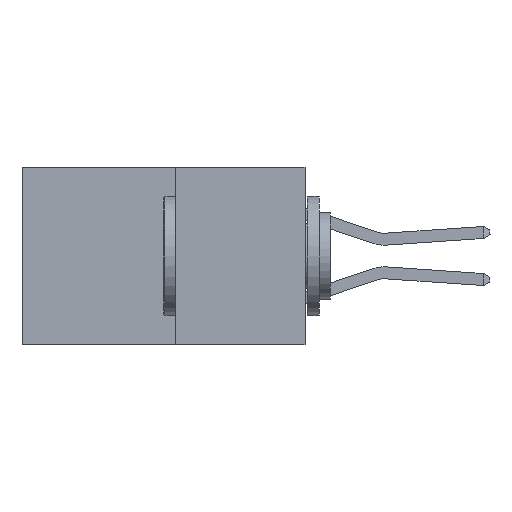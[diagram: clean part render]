
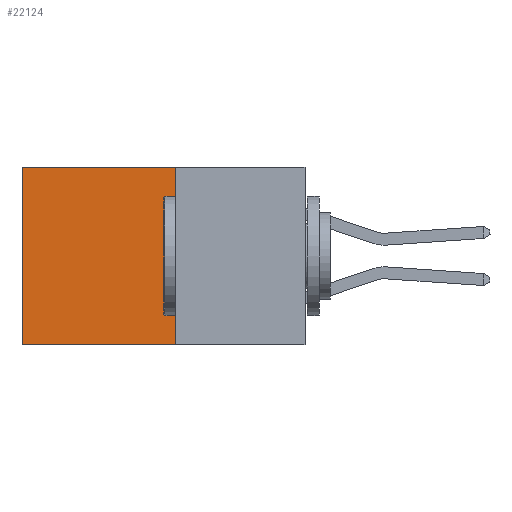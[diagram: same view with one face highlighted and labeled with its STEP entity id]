
A CAD part, left-side view. The second image highlights one B-rep face of the part: STEP entity #22124.
In plain terms, the highlighted planar face has unit normal (-1, 0, 0).
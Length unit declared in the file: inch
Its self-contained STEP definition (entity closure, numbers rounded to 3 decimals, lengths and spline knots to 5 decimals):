
#826 = CARTESIAN_POINT ( 'NONE',  ( 0.277, 0.59, -0.37 ) ) ;
#838 = VECTOR ( 'NONE', #5573, 39.37008 ) ;
#1346 = AXIS2_PLACEMENT_3D ( 'NONE', #10093, #24088, #12134 ) ;
#1843 = PLANE ( 'NONE',  #1346 ) ;
#1901 = EDGE_CURVE ( 'NONE', #25832, #14710, #22952, .T. ) ;
#1907 = EDGE_CURVE ( 'NONE', #25832, #2694, #22337, .T. ) ;
#2694 = VERTEX_POINT ( 'NONE', #5065 ) ;
#2877 = DIRECTION ( 'NONE',  ( 0., 0., -1. ) ) ;
#5065 = CARTESIAN_POINT ( 'NONE',  ( 0.277, 0.27, -0.37 ) ) ;
#5432 = ORIENTED_EDGE ( 'NONE', *, *, #14664, .F. ) ;
#5573 = DIRECTION ( 'NONE',  ( 0., 0., -1. ) ) ;
#5765 = DIRECTION ( 'NONE',  ( 0., 1., 0. ) ) ;
#6610 = CARTESIAN_POINT ( 'NONE',  ( 0.277, 0.27, 0. ) ) ;
#6924 = VECTOR ( 'NONE', #5765, 39.37008 ) ;
#8030 = LINE ( 'NONE', #826, #18157 ) ;
#9894 = CARTESIAN_POINT ( 'NONE',  ( 0.277, 0.27, -0.37 ) ) ;
#10093 = CARTESIAN_POINT ( 'NONE',  ( 0.277, 0.27, -0.37 ) ) ;
#10133 = ORIENTED_EDGE ( 'NONE', *, *, #1901, .T. ) ;
#10216 = DIRECTION ( 'NONE',  ( 0., 1., 0. ) ) ;
#12134 = DIRECTION ( 'NONE',  ( 0., 0., -1. ) ) ;
#12203 = CARTESIAN_POINT ( 'NONE',  ( 0.277, 0.27, 0. ) ) ;
#13192 = EDGE_LOOP ( 'NONE', ( #24089, #5432, #23364, #10133 ) ) ;
#14034 = CARTESIAN_POINT ( 'NONE',  ( 0.277, 0.59, -0.37 ) ) ;
#14457 = CARTESIAN_POINT ( 'NONE',  ( 0.277, 0.59, 0. ) ) ;
#14664 = EDGE_CURVE ( 'NONE', #2694, #20780, #15214, .T. ) ;
#14710 = VERTEX_POINT ( 'NONE', #14457 ) ;
#15214 = LINE ( 'NONE', #24207, #19893 ) ;
#16355 = EDGE_CURVE ( 'NONE', #14710, #20780, #8030, .T. ) ;
#18157 = VECTOR ( 'NONE', #2877, 39.37008 ) ;
#19893 = VECTOR ( 'NONE', #10216, 39.37008 ) ;
#20780 = VERTEX_POINT ( 'NONE', #14034 ) ;
#22124 = ADVANCED_FACE ( 'NONE', ( #25585 ), #1843, .F. ) ;
#22337 = LINE ( 'NONE', #9894, #838 ) ;
#22952 = LINE ( 'NONE', #12203, #6924 ) ;
#23364 = ORIENTED_EDGE ( 'NONE', *, *, #1907, .F. ) ;
#24088 = DIRECTION ( 'NONE',  ( 1., 0., 0. ) ) ;
#24089 = ORIENTED_EDGE ( 'NONE', *, *, #16355, .T. ) ;
#24207 = CARTESIAN_POINT ( 'NONE',  ( 0.277, 0.27, -0.37 ) ) ;
#25585 = FACE_OUTER_BOUND ( 'NONE', #13192, .T. ) ;
#25832 = VERTEX_POINT ( 'NONE', #6610 ) ;
